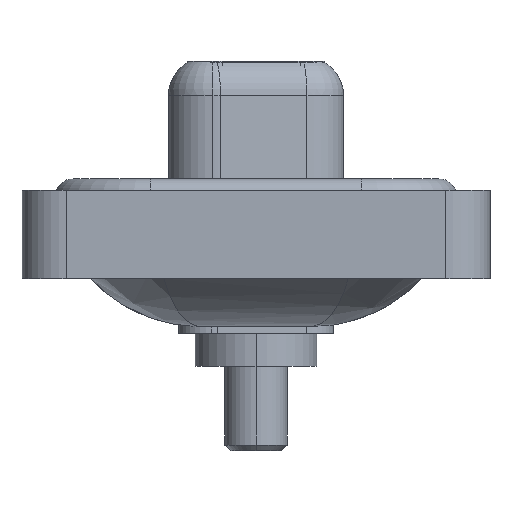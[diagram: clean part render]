
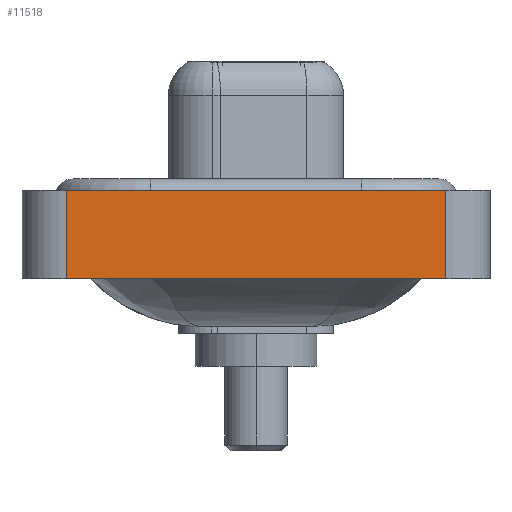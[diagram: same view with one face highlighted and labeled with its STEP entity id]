
A CAD part, left-side view. The second image highlights one B-rep face of the part: STEP entity #11518.
In plain terms, the highlighted planar face has unit normal (-1, 0, 0).
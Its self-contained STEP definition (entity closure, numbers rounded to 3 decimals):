
#321 = ORIENTED_EDGE ( 'NONE', *, *, #16274, .T. ) ;
#1205 = VECTOR ( 'NONE', #8861, 1000. ) ;
#2257 = LINE ( 'NONE', #11419, #4656 ) ;
#2476 = DIRECTION ( 'NONE',  ( 0., 0., 1. ) ) ;
#2489 = EDGE_CURVE ( 'NONE', #6927, #13081, #2257, .T. ) ;
#2503 = EDGE_CURVE ( 'NONE', #3409, #3366, #15713, .T. ) ;
#2524 = DIRECTION ( 'NONE',  ( 0., -1., 0. ) ) ;
#3366 = VERTEX_POINT ( 'NONE', #16276 ) ;
#3384 = DIRECTION ( 'NONE',  ( 0., 0., 1. ) ) ;
#3409 = VERTEX_POINT ( 'NONE', #16864 ) ;
#3627 = CARTESIAN_POINT ( 'NONE',  ( -7.25, -8.55, -3.6 ) ) ;
#3753 = FACE_OUTER_BOUND ( 'NONE', #14005, .T. ) ;
#3838 = VECTOR ( 'NONE', #2524, 1000. ) ;
#4656 = VECTOR ( 'NONE', #13742, 1000. ) ;
#5853 = LINE ( 'NONE', #16231, #15488 ) ;
#6282 = CARTESIAN_POINT ( 'NONE',  ( -7.25, -8.55, -3.6 ) ) ;
#6915 = AXIS2_PLACEMENT_3D ( 'NONE', #14038, #11375, #2476 ) ;
#6927 = VERTEX_POINT ( 'NONE', #13486 ) ;
#7603 = PLANE ( 'NONE',  #6915 ) ;
#7823 = CARTESIAN_POINT ( 'NONE',  ( -7.25, -8.55, 0.4 ) ) ;
#8861 = DIRECTION ( 'NONE',  ( 0., 0., 1. ) ) ;
#10240 = EDGE_CURVE ( 'NONE', #6927, #3409, #5853, .T. ) ;
#11375 = DIRECTION ( 'NONE',  ( -1., 0., 0. ) ) ;
#11419 = CARTESIAN_POINT ( 'NONE',  ( -7.25, -8.55, -3.6 ) ) ;
#11518 = ADVANCED_FACE ( 'NONE', ( #3753 ), #7603, .T. ) ;
#11738 = ORIENTED_EDGE ( 'NONE', *, *, #2489, .T. ) ;
#12980 = ORIENTED_EDGE ( 'NONE', *, *, #2503, .F. ) ;
#13081 = VERTEX_POINT ( 'NONE', #6282 ) ;
#13486 = CARTESIAN_POINT ( 'NONE',  ( -7.25, 8.55, -3.6 ) ) ;
#13742 = DIRECTION ( 'NONE',  ( 0., -1., 0. ) ) ;
#13915 = ORIENTED_EDGE ( 'NONE', *, *, #10240, .F. ) ;
#14005 = EDGE_LOOP ( 'NONE', ( #321, #12980, #13915, #11738 ) ) ;
#14038 = CARTESIAN_POINT ( 'NONE',  ( -7.25, -8.55, -3.6 ) ) ;
#15488 = VECTOR ( 'NONE', #3384, 1000. ) ;
#15713 = LINE ( 'NONE', #7823, #3838 ) ;
#16231 = CARTESIAN_POINT ( 'NONE',  ( -7.25, 8.55, -3.6 ) ) ;
#16274 = EDGE_CURVE ( 'NONE', #13081, #3366, #16730, .T. ) ;
#16276 = CARTESIAN_POINT ( 'NONE',  ( -7.25, -8.55, 0.4 ) ) ;
#16730 = LINE ( 'NONE', #3627, #1205 ) ;
#16864 = CARTESIAN_POINT ( 'NONE',  ( -7.25, 8.55, 0.4 ) ) ;
